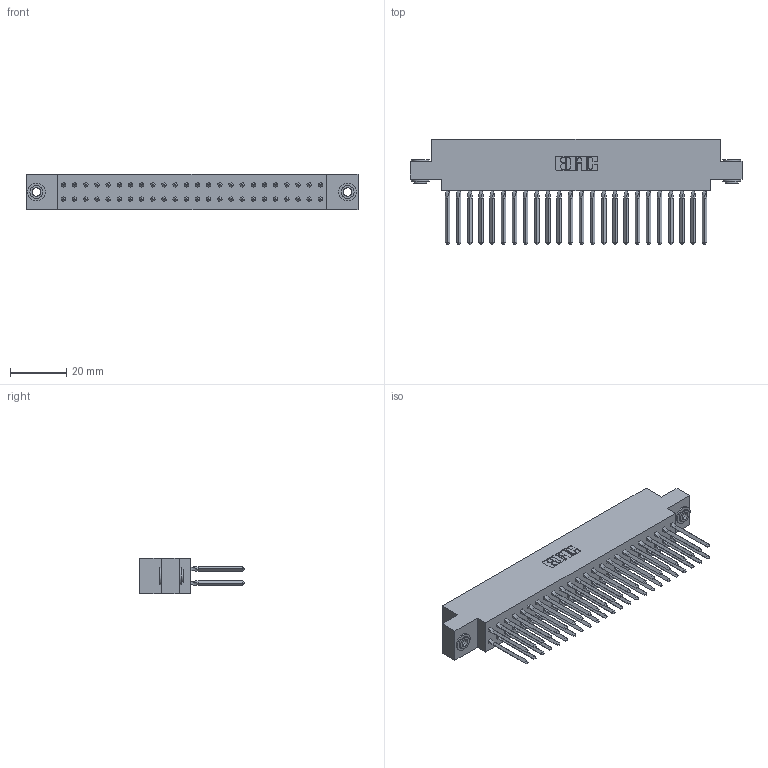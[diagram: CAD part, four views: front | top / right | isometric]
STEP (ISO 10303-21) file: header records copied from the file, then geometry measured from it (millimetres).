
FILE_DESCRIPTION (( 'STEP AP203' ), '1' );
FILE_NAME ('317-048-542-803.STEP', '2020-02-28T02:48:59', ( '' ), ( '' ), 'SwSTEP 2.0', 'SolidWorks 2016', '' );
FILE_SCHEMA (( 'CONFIG_CONTROL_DESIGN' ));
Length unit declared in the file: inch
Products named in the file (4): 345-250-002_345-250-002-102; 317-290-003_542; 317 Part_.156 Dia - TH; 317-048-542-803
Assembly tree (51 placements, depth 2):
  317-048-542-803
    317 Part_.156 Dia - TH
    317-290-003_542  x48
    345-250-002_345-250-002-102  x2
Bounding box: 117.81 x 37.34 x 12.7 mm (x, y, z)
Volume: 18740.8 mm3; surface area: 25699.4 mm2
Topology: 51 solids, 51 shells, 2876 faces, 8031 edges, 5126 vertices
Faces by surface type: plane 2276, cylinder 400, bspline 192, cone 8
Entity records: 36870 total; most frequent: CARTESIAN_POINT 6648, ORIENTED_EDGE 6304, DIRECTION 5374, EDGE_CURVE 3152, VECTOR 2958, LINE 2958, VERTEX_POINT 2094, AXIS2_PLACEMENT_3D 1208
